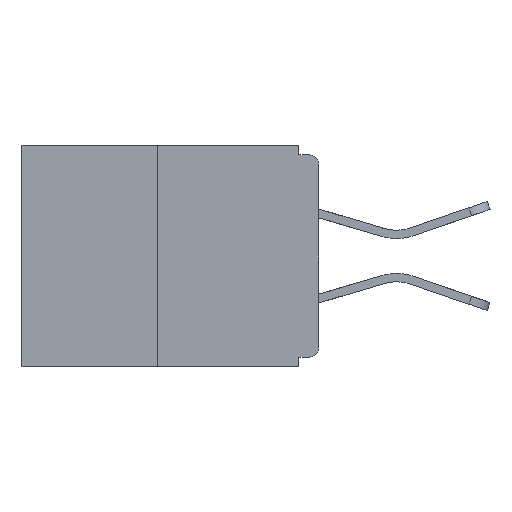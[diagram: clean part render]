
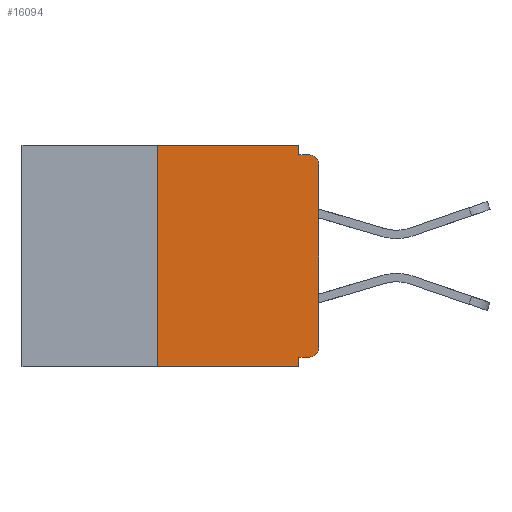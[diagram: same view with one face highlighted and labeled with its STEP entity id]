
A CAD part, left-side view. The second image highlights one B-rep face of the part: STEP entity #16094.
In plain terms, the highlighted planar face has unit normal (-1, 0, 0).
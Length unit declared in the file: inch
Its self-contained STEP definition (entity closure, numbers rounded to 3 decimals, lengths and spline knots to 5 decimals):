
#704 = EDGE_CURVE ( 'NONE', #6957, #10162, #3136, .T. ) ;
#892 = AXIS2_PLACEMENT_3D ( 'NONE', #6561, #19449, #9677 ) ;
#1947 = ORIENTED_EDGE ( 'NONE', *, *, #10333, .T. ) ;
#1961 = DIRECTION ( 'NONE',  ( 0., 0., 1. ) ) ;
#2054 = VERTEX_POINT ( 'NONE', #8585 ) ;
#2126 = DIRECTION ( 'NONE',  ( 1., 0., 0. ) ) ;
#2348 = VERTEX_POINT ( 'NONE', #11037 ) ;
#2726 = CARTESIAN_POINT ( 'NONE',  ( 0., 0.25, -0.343 ) ) ;
#3136 = LINE ( 'NONE', #14912, #17141 ) ;
#3191 = DIRECTION ( 'NONE',  ( 0., -1., 0. ) ) ;
#3222 = CARTESIAN_POINT ( 'NONE',  ( 0., 0.015, -0.015 ) ) ;
#3437 = EDGE_CURVE ( 'NONE', #9549, #17752, #13959, .T. ) ;
#3920 = DIRECTION ( 'NONE',  ( -1., 0., 0. ) ) ;
#4005 = LINE ( 'NONE', #7332, #18498 ) ;
#4251 = VERTEX_POINT ( 'NONE', #3222 ) ;
#4749 = EDGE_CURVE ( 'NONE', #11573, #6957, #11168, .T. ) ;
#4941 = LINE ( 'NONE', #14720, #13538 ) ;
#5108 = DIRECTION ( 'NONE',  ( 0., 0., 1. ) ) ;
#5226 = CARTESIAN_POINT ( 'NONE',  ( 0., 0.031, 0. ) ) ;
#5779 = ORIENTED_EDGE ( 'NONE', *, *, #8568, .F. ) ;
#5970 = DIRECTION ( 'NONE',  ( 0., -1., 0. ) ) ;
#6154 = LINE ( 'NONE', #20996, #11465 ) ;
#6561 = CARTESIAN_POINT ( 'NONE',  ( 0., 0.015, -0.313 ) ) ;
#6797 = CARTESIAN_POINT ( 'NONE',  ( 0., 0., -0.313 ) ) ;
#6826 = ORIENTED_EDGE ( 'NONE', *, *, #704, .T. ) ;
#6957 = VERTEX_POINT ( 'NONE', #6797 ) ;
#7103 = ORIENTED_EDGE ( 'NONE', *, *, #12734, .T. ) ;
#7185 = ORIENTED_EDGE ( 'NONE', *, *, #15676, .F. ) ;
#7332 = CARTESIAN_POINT ( 'NONE',  ( 0., 0.46, -0.343 ) ) ;
#7801 = DIRECTION ( 'NONE',  ( 0., 1., 0. ) ) ;
#8357 = VERTEX_POINT ( 'NONE', #2726 ) ;
#8547 = LINE ( 'NONE', #16172, #18737 ) ;
#8568 = EDGE_CURVE ( 'NONE', #2348, #2054, #13823, .T. ) ;
#8585 = CARTESIAN_POINT ( 'NONE',  ( 0., 0.031, -0.343 ) ) ;
#9226 = VERTEX_POINT ( 'NONE', #20653 ) ;
#9549 = VERTEX_POINT ( 'NONE', #5226 ) ;
#9651 = VECTOR ( 'NONE', #11654, 39.37008 ) ;
#9677 = DIRECTION ( 'NONE',  ( 0., 0., -1. ) ) ;
#9840 = DIRECTION ( 'NONE',  ( 0., 0., -1. ) ) ;
#10162 = VERTEX_POINT ( 'NONE', #18448 ) ;
#10333 = EDGE_CURVE ( 'NONE', #10162, #4251, #19359, .T. ) ;
#10385 = ORIENTED_EDGE ( 'NONE', *, *, #12957, .F. ) ;
#11037 = CARTESIAN_POINT ( 'NONE',  ( 0., 0.031, -0.328 ) ) ;
#11168 = CIRCLE ( 'NONE', #892, 0.015 ) ;
#11258 = FACE_OUTER_BOUND ( 'NONE', #18621, .T. ) ;
#11447 = CARTESIAN_POINT ( 'NONE',  ( 0., 0.031, 0. ) ) ;
#11465 = VECTOR ( 'NONE', #3191, 39.37008 ) ;
#11541 = CARTESIAN_POINT ( 'NONE',  ( 0., 0.031, -0.343 ) ) ;
#11573 = VERTEX_POINT ( 'NONE', #11833 ) ;
#11654 = DIRECTION ( 'NONE',  ( 0., 0., -1. ) ) ;
#11833 = CARTESIAN_POINT ( 'NONE',  ( 0., 0.015, -0.328 ) ) ;
#12247 = CARTESIAN_POINT ( 'NONE',  ( 0., 0.015, -0.03 ) ) ;
#12443 = ORIENTED_EDGE ( 'NONE', *, *, #14946, .F. ) ;
#12734 = EDGE_CURVE ( 'NONE', #8357, #2054, #4005, .T. ) ;
#12769 = CARTESIAN_POINT ( 'NONE',  ( 0., 0.031, -0.015 ) ) ;
#12957 = EDGE_CURVE ( 'NONE', #8357, #9226, #8547, .T. ) ;
#13538 = VECTOR ( 'NONE', #16297, 39.37008 ) ;
#13811 = DIRECTION ( 'NONE',  ( 0., 0., -1. ) ) ;
#13823 = LINE ( 'NONE', #11541, #19476 ) ;
#13959 = LINE ( 'NONE', #11447, #9651 ) ;
#14400 = ORIENTED_EDGE ( 'NONE', *, *, #4749, .T. ) ;
#14484 = LINE ( 'NONE', #17672, #16294 ) ;
#14720 = CARTESIAN_POINT ( 'NONE',  ( 0., 0.46, 0. ) ) ;
#14912 = CARTESIAN_POINT ( 'NONE',  ( 0., 0., 0. ) ) ;
#14946 = EDGE_CURVE ( 'NONE', #9226, #9549, #4941, .T. ) ;
#15061 = AXIS2_PLACEMENT_3D ( 'NONE', #18367, #2126, #16792 ) ;
#15676 = EDGE_CURVE ( 'NONE', #11573, #2348, #14484, .T. ) ;
#15678 = AXIS2_PLACEMENT_3D ( 'NONE', #12247, #3920, #13811 ) ;
#16094 = ADVANCED_FACE ( 'NONE', ( #11258 ), #16584, .F. ) ;
#16172 = CARTESIAN_POINT ( 'NONE',  ( 0., 0.25, 0. ) ) ;
#16193 = ORIENTED_EDGE ( 'NONE', *, *, #3437, .F. ) ;
#16294 = VECTOR ( 'NONE', #7801, 39.37008 ) ;
#16297 = DIRECTION ( 'NONE',  ( 0., -1., 0. ) ) ;
#16584 = PLANE ( 'NONE',  #15061 ) ;
#16792 = DIRECTION ( 'NONE',  ( 0., 0., -1. ) ) ;
#17141 = VECTOR ( 'NONE', #5108, 39.37008 ) ;
#17672 = CARTESIAN_POINT ( 'NONE',  ( 0., 0., -0.328 ) ) ;
#17752 = VERTEX_POINT ( 'NONE', #12769 ) ;
#17958 = EDGE_CURVE ( 'NONE', #17752, #4251, #6154, .T. ) ;
#18367 = CARTESIAN_POINT ( 'NONE',  ( 0., 0.46, 0. ) ) ;
#18448 = CARTESIAN_POINT ( 'NONE',  ( 0., 0., -0.03 ) ) ;
#18498 = VECTOR ( 'NONE', #5970, 39.37008 ) ;
#18621 = EDGE_LOOP ( 'NONE', ( #12443, #10385, #7103, #5779, #7185, #14400, #6826, #1947, #19177, #16193 ) ) ;
#18737 = VECTOR ( 'NONE', #1961, 39.37008 ) ;
#19177 = ORIENTED_EDGE ( 'NONE', *, *, #17958, .F. ) ;
#19359 = CIRCLE ( 'NONE', #15678, 0.015 ) ;
#19449 = DIRECTION ( 'NONE',  ( -1., 0., 0. ) ) ;
#19476 = VECTOR ( 'NONE', #9840, 39.37008 ) ;
#20653 = CARTESIAN_POINT ( 'NONE',  ( 0., 0.25, 0. ) ) ;
#20996 = CARTESIAN_POINT ( 'NONE',  ( 0., 0., -0.015 ) ) ;
